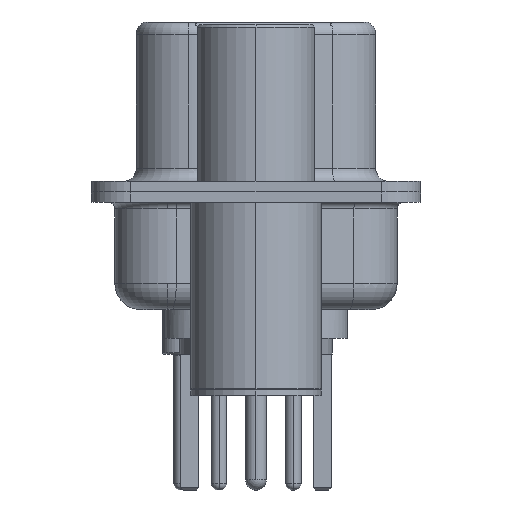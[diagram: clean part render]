
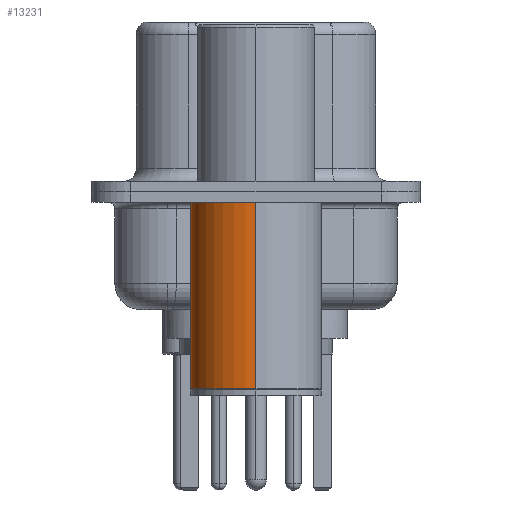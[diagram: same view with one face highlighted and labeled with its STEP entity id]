
A CAD part, left-side view. The second image highlights one B-rep face of the part: STEP entity #13231.
In plain terms, the highlighted cylindrical face has radius 2.5 mm (diameter 5 mm), a partial arc.
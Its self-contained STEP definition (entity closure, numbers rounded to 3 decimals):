
#1409 = CARTESIAN_POINT ( 'NONE',  ( 0., 0., -0.4 ) ) ;
#2235 = FACE_OUTER_BOUND ( 'NONE', #21849, .T. ) ;
#3323 = AXIS2_PLACEMENT_3D ( 'NONE', #16461, #7235, #23420 ) ;
#4595 = LINE ( 'NONE', #5674, #11374 ) ;
#4631 = EDGE_CURVE ( 'NONE', #23474, #13964, #12830, .T. ) ;
#4956 = CARTESIAN_POINT ( 'NONE',  ( 2.5, 0., -7.525 ) ) ;
#5674 = CARTESIAN_POINT ( 'NONE',  ( -2.5, 0., 0.581 ) ) ;
#6454 = EDGE_CURVE ( 'NONE', #18240, #23474, #16817, .T. ) ;
#7235 = DIRECTION ( 'NONE',  ( 0., 0., 1. ) ) ;
#7767 = DIRECTION ( 'NONE',  ( 1., 0., 0. ) ) ;
#8230 = DIRECTION ( 'NONE',  ( 0., 0., 1. ) ) ;
#8234 = CARTESIAN_POINT ( 'NONE',  ( -2.5, 0., -7.525 ) ) ;
#9351 = ORIENTED_EDGE ( 'NONE', *, *, #4631, .F. ) ;
#11374 = VECTOR ( 'NONE', #21825, 1000. ) ;
#12795 = DIRECTION ( 'NONE',  ( 0., 0., 1. ) ) ;
#12830 = CIRCLE ( 'NONE', #21854, 2.5 ) ;
#12850 = CIRCLE ( 'NONE', #16813, 2.5 ) ;
#13197 = CARTESIAN_POINT ( 'NONE',  ( 2.5, 0., 0.581 ) ) ;
#13231 = ADVANCED_FACE ( 'NONE', ( #2235 ), #18441, .T. ) ;
#13964 = VERTEX_POINT ( 'NONE', #21263 ) ;
#15000 = EDGE_CURVE ( 'NONE', #18240, #16128, #12850, .T. ) ;
#15327 = VECTOR ( 'NONE', #12795, 1000. ) ;
#15816 = ORIENTED_EDGE ( 'NONE', *, *, #6454, .F. ) ;
#16128 = VERTEX_POINT ( 'NONE', #8234 ) ;
#16461 = CARTESIAN_POINT ( 'NONE',  ( 0., 0., 0.581 ) ) ;
#16813 = AXIS2_PLACEMENT_3D ( 'NONE', #22116, #8230, #24457 ) ;
#16817 = LINE ( 'NONE', #13197, #15327 ) ;
#18240 = VERTEX_POINT ( 'NONE', #4956 ) ;
#18441 = CYLINDRICAL_SURFACE ( 'NONE', #3323, 2.5 ) ;
#18573 = CARTESIAN_POINT ( 'NONE',  ( 2.5, 0., -0.4 ) ) ;
#21115 = DIRECTION ( 'NONE',  ( 0., 0., 1. ) ) ;
#21263 = CARTESIAN_POINT ( 'NONE',  ( -2.5, 0., -0.4 ) ) ;
#21668 = ORIENTED_EDGE ( 'NONE', *, *, #24897, .T. ) ;
#21825 = DIRECTION ( 'NONE',  ( 0., 0., 1. ) ) ;
#21849 = EDGE_LOOP ( 'NONE', ( #28227, #21668, #9351, #15816 ) ) ;
#21854 = AXIS2_PLACEMENT_3D ( 'NONE', #1409, #21115, #7767 ) ;
#22116 = CARTESIAN_POINT ( 'NONE',  ( 0., 0., -7.525 ) ) ;
#23420 = DIRECTION ( 'NONE',  ( 1., 0., 0. ) ) ;
#23474 = VERTEX_POINT ( 'NONE', #18573 ) ;
#24457 = DIRECTION ( 'NONE',  ( 1., 0., 0. ) ) ;
#24897 = EDGE_CURVE ( 'NONE', #16128, #13964, #4595, .T. ) ;
#28227 = ORIENTED_EDGE ( 'NONE', *, *, #15000, .T. ) ;
